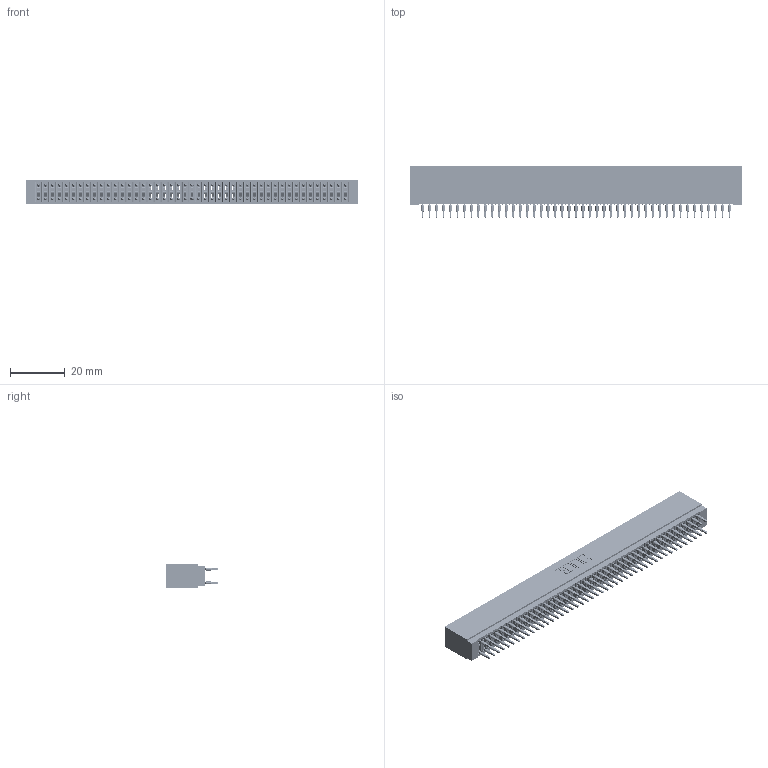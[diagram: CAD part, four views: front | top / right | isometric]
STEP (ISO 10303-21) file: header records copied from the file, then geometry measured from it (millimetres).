
FILE_DESCRIPTION (( 'STEP AP203' ), '1' );
FILE_NAME ('725-090-560-201.STEP', '2026-02-24T19:31:15', ( '' ), ( '' ), 'SwSTEP 2.0', 'SolidWorks 2023', '' );
FILE_SCHEMA (( 'CONFIG_CONTROL_DESIGN' ));
Length unit declared in the file: millimetre
Products named in the file (3): 725-090-560-201; 745-292-001_560; 725 Part_Insulator Option - 01
Assembly tree (91 placements, depth 2):
  725-090-560-201
    725 Part_Insulator Option - 01
    745-292-001_560  x90
Bounding box: 120.9 x 18.8 x 8.89 mm (x, y, z)
Volume: 9905.2 mm3; surface area: 22404.2 mm2
Topology: 91 solids, 91 shells, 8960 faces, 24509 edges, 15558 vertices
Faces by surface type: plane 4645, cylinder 1975, bspline 1800, torus 540
Entity records: 75636 total; most frequent: CARTESIAN_POINT 13621, ORIENTED_EDGE 13062, DIRECTION 11415, EDGE_CURVE 6531, LINE 6071, VECTOR 6071, VERTEX_POINT 4166, AXIS2_PLACEMENT_3D 2672
